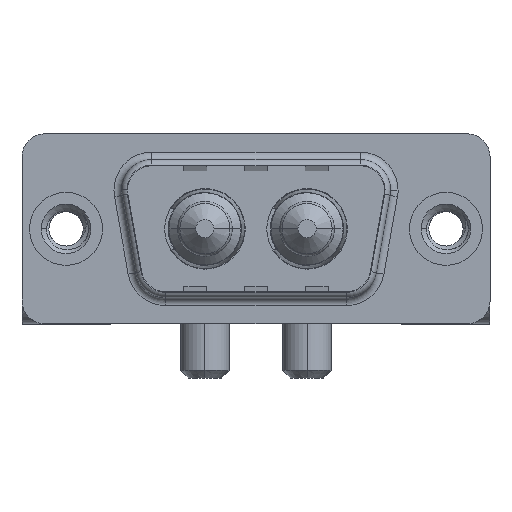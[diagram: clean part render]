
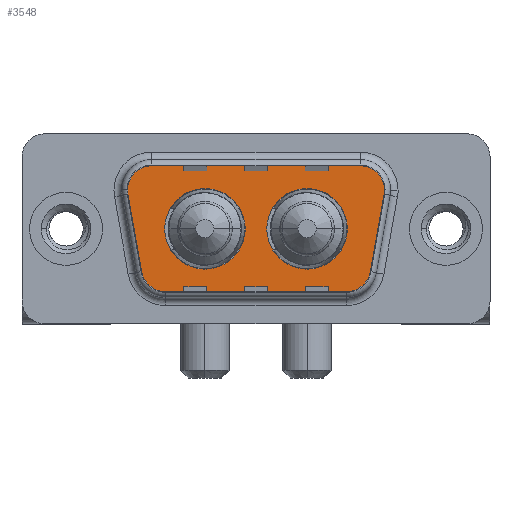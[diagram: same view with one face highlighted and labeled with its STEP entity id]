
A CAD part, top view. The second image highlights one B-rep face of the part: STEP entity #3548.
In plain terms, the highlighted planar face has unit normal (0, 0, 1).
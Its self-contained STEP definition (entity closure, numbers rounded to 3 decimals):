
#85 = CARTESIAN_POINT ( 'NONE',  ( 9.14, 0., 0. ) ) ;
#160 = ORIENTED_EDGE ( 'NONE', *, *, #9335, .T. ) ;
#173 = CARTESIAN_POINT ( 'NONE',  ( 6.459, -2.9, 0. ) ) ;
#208 = ORIENTED_EDGE ( 'NONE', *, *, #1966, .T. ) ;
#296 = CARTESIAN_POINT ( 'NONE',  ( 18.541, -2.9, 0. ) ) ;
#370 = ORIENTED_EDGE ( 'NONE', *, *, #9653, .T. ) ;
#516 = CARTESIAN_POINT ( 'NONE',  ( 3.466, 2.553, 0. ) ) ;
#538 = LINE ( 'NONE', #2681, #9395 ) ;
#579 = DIRECTION ( 'NONE',  ( 1., 0., 0. ) ) ;
#612 = AXIS2_PLACEMENT_3D ( 'NONE', #296, #8820, #9711 ) ;
#729 = ORIENTED_EDGE ( 'NONE', *, *, #10192, .F. ) ;
#896 = CARTESIAN_POINT ( 'NONE',  ( 19.564, 2.9, 0. ) ) ;
#977 = EDGE_CURVE ( 'NONE', #6027, #11507, #538, .T. ) ;
#1020 = CARTESIAN_POINT ( 'NONE',  ( 5.436, 4.9, 0. ) ) ;
#1031 = CARTESIAN_POINT ( 'NONE',  ( 19.564, 2.9, 0. ) ) ;
#1094 = ORIENTED_EDGE ( 'NONE', *, *, #4804, .F. ) ;
#1356 = DIRECTION ( 'NONE',  ( 1., 0., 0. ) ) ;
#1407 = CIRCLE ( 'NONE', #4452, 2. ) ;
#1592 = VERTEX_POINT ( 'NONE', #5201 ) ;
#1645 = PLANE ( 'NONE',  #7467 ) ;
#1786 = CARTESIAN_POINT ( 'NONE',  ( 5.436, 4.9, 0. ) ) ;
#1832 = DIRECTION ( 'NONE',  ( -1., 0., 0. ) ) ;
#1966 = EDGE_CURVE ( 'NONE', #10022, #3323, #4750, .T. ) ;
#1969 = CARTESIAN_POINT ( 'NONE',  ( 11.79, 0., 0. ) ) ;
#2035 = AXIS2_PLACEMENT_3D ( 'NONE', #9243, #6271, #7282 ) ;
#2036 = DIRECTION ( 'NONE',  ( -1., 0., 0. ) ) ;
#2100 = VERTEX_POINT ( 'NONE', #7900 ) ;
#2272 = VERTEX_POINT ( 'NONE', #10055 ) ;
#2318 = VERTEX_POINT ( 'NONE', #4304 ) ;
#2591 = FACE_BOUND ( 'NONE', #4614, .T. ) ;
#2600 = EDGE_LOOP ( 'NONE', ( #5776, #1094 ) ) ;
#2681 = CARTESIAN_POINT ( 'NONE',  ( 21.534, 2.553, 0. ) ) ;
#2705 = LINE ( 'NONE', #11487, #9283 ) ;
#3005 = DIRECTION ( 'NONE',  ( 0., 0., 1. ) ) ;
#3055 = CIRCLE ( 'NONE', #8319, 2.65 ) ;
#3077 = DIRECTION ( 'NONE',  ( -1., 0., 0. ) ) ;
#3105 = ORIENTED_EDGE ( 'NONE', *, *, #7557, .T. ) ;
#3113 = ORIENTED_EDGE ( 'NONE', *, *, #12267, .T. ) ;
#3160 = ORIENTED_EDGE ( 'NONE', *, *, #11364, .T. ) ;
#3323 = VERTEX_POINT ( 'NONE', #1786 ) ;
#3409 = LINE ( 'NONE', #516, #6702 ) ;
#3548 = ADVANCED_FACE ( 'NONE', ( #8413, #2591, #12083 ), #1645, .T. ) ;
#3656 = AXIS2_PLACEMENT_3D ( 'NONE', #11680, #3005, #6863 ) ;
#3727 = VECTOR ( 'NONE', #8730, 1000. ) ;
#3822 = CIRCLE ( 'NONE', #8668, 2. ) ;
#3905 = DIRECTION ( 'NONE',  ( 0., 0., 1. ) ) ;
#4198 = VERTEX_POINT ( 'NONE', #8765 ) ;
#4213 = EDGE_CURVE ( 'NONE', #10918, #2272, #7889, .T. ) ;
#4224 = EDGE_CURVE ( 'NONE', #5443, #2100, #8508, .T. ) ;
#4304 = CARTESIAN_POINT ( 'NONE',  ( 21.564, 2.9, 0. ) ) ;
#4452 = AXIS2_PLACEMENT_3D ( 'NONE', #5507, #10253, #579 ) ;
#4614 = EDGE_LOOP ( 'NONE', ( #9905, #729 ) ) ;
#4750 = LINE ( 'NONE', #1020, #3727 ) ;
#4804 = EDGE_CURVE ( 'NONE', #2100, #5443, #3055, .T. ) ;
#5037 = CIRCLE ( 'NONE', #612, 2. ) ;
#5201 = CARTESIAN_POINT ( 'NONE',  ( 6.49, 0., 0. ) ) ;
#5383 = CIRCLE ( 'NONE', #5595, 2. ) ;
#5443 = VERTEX_POINT ( 'NONE', #5802 ) ;
#5507 = CARTESIAN_POINT ( 'NONE',  ( 5.436, 2.9, 0. ) ) ;
#5549 = DIRECTION ( 'NONE',  ( 1., 0., 0. ) ) ;
#5595 = AXIS2_PLACEMENT_3D ( 'NONE', #896, #8595, #1832 ) ;
#5776 = ORIENTED_EDGE ( 'NONE', *, *, #4224, .F. ) ;
#5802 = CARTESIAN_POINT ( 'NONE',  ( 18.51, 0., 0. ) ) ;
#6027 = VERTEX_POINT ( 'NONE', #7836 ) ;
#6159 = EDGE_LOOP ( 'NONE', ( #8062, #10809, #3113, #160, #208, #370, #3105, #9988, #3160 ) ) ;
#6271 = DIRECTION ( 'NONE',  ( 0., 0., 1. ) ) ;
#6540 = DIRECTION ( 'NONE',  ( 0.174, 0.985, 0. ) ) ;
#6647 = DIRECTION ( 'NONE',  ( 0., 0., 1. ) ) ;
#6702 = VECTOR ( 'NONE', #11132, 1000. ) ;
#6863 = DIRECTION ( 'NONE',  ( 1., 0., 0. ) ) ;
#7103 = CARTESIAN_POINT ( 'NONE',  ( 15.86, 0., 0. ) ) ;
#7193 = VERTEX_POINT ( 'NONE', #1969 ) ;
#7207 = VERTEX_POINT ( 'NONE', #10690 ) ;
#7209 = EDGE_CURVE ( 'NONE', #7193, #1592, #12160, .T. ) ;
#7282 = DIRECTION ( 'NONE',  ( 1., 0., 0. ) ) ;
#7301 = AXIS2_PLACEMENT_3D ( 'NONE', #85, #6647, #9749 ) ;
#7467 = AXIS2_PLACEMENT_3D ( 'NONE', #11130, #9227, #9358 ) ;
#7557 = EDGE_CURVE ( 'NONE', #4198, #10918, #3409, .T. ) ;
#7836 = CARTESIAN_POINT ( 'NONE',  ( 20.511, -3.247, 0. ) ) ;
#7889 = CIRCLE ( 'NONE', #9105, 2. ) ;
#7900 = CARTESIAN_POINT ( 'NONE',  ( 13.21, 0., 0. ) ) ;
#8062 = ORIENTED_EDGE ( 'NONE', *, *, #11552, .T. ) ;
#8319 = AXIS2_PLACEMENT_3D ( 'NONE', #7103, #10021, #1356 ) ;
#8413 = FACE_BOUND ( 'NONE', #2600, .T. ) ;
#8508 = CIRCLE ( 'NONE', #3656, 2.65 ) ;
#8595 = DIRECTION ( 'NONE',  ( 0., 0., 1. ) ) ;
#8668 = AXIS2_PLACEMENT_3D ( 'NONE', #1031, #11651, #2036 ) ;
#8730 = DIRECTION ( 'NONE',  ( -1., 0., 0. ) ) ;
#8765 = CARTESIAN_POINT ( 'NONE',  ( 3.466, 2.553, 0. ) ) ;
#8820 = DIRECTION ( 'NONE',  ( 0., 0., 1. ) ) ;
#9105 = AXIS2_PLACEMENT_3D ( 'NONE', #173, #3905, #3077 ) ;
#9227 = DIRECTION ( 'NONE',  ( 0., 0., 1. ) ) ;
#9243 = CARTESIAN_POINT ( 'NONE',  ( 9.14, 0., 0. ) ) ;
#9283 = VECTOR ( 'NONE', #5549, 1000. ) ;
#9297 = CIRCLE ( 'NONE', #2035, 2.65 ) ;
#9335 = EDGE_CURVE ( 'NONE', #2318, #10022, #3822, .T. ) ;
#9358 = DIRECTION ( 'NONE',  ( 1., 0., 0. ) ) ;
#9395 = VECTOR ( 'NONE', #6540, 1000. ) ;
#9546 = CARTESIAN_POINT ( 'NONE',  ( 4.489, -3.247, 0. ) ) ;
#9653 = EDGE_CURVE ( 'NONE', #3323, #4198, #1407, .T. ) ;
#9711 = DIRECTION ( 'NONE',  ( 1., 0., 0. ) ) ;
#9749 = DIRECTION ( 'NONE',  ( 1., 0., 0. ) ) ;
#9905 = ORIENTED_EDGE ( 'NONE', *, *, #7209, .F. ) ;
#9988 = ORIENTED_EDGE ( 'NONE', *, *, #4213, .T. ) ;
#10021 = DIRECTION ( 'NONE',  ( 0., 0., 1. ) ) ;
#10022 = VERTEX_POINT ( 'NONE', #11908 ) ;
#10055 = CARTESIAN_POINT ( 'NONE',  ( 6.459, -4.9, 0. ) ) ;
#10192 = EDGE_CURVE ( 'NONE', #1592, #7193, #9297, .T. ) ;
#10253 = DIRECTION ( 'NONE',  ( 0., 0., 1. ) ) ;
#10690 = CARTESIAN_POINT ( 'NONE',  ( 18.541, -4.9, 0. ) ) ;
#10809 = ORIENTED_EDGE ( 'NONE', *, *, #977, .T. ) ;
#10918 = VERTEX_POINT ( 'NONE', #9546 ) ;
#11130 = CARTESIAN_POINT ( 'NONE',  ( 18.541, -2.9, 0. ) ) ;
#11132 = DIRECTION ( 'NONE',  ( 0.174, -0.985, 0. ) ) ;
#11364 = EDGE_CURVE ( 'NONE', #2272, #7207, #2705, .T. ) ;
#11487 = CARTESIAN_POINT ( 'NONE',  ( 6.459, -4.9, 0. ) ) ;
#11507 = VERTEX_POINT ( 'NONE', #11809 ) ;
#11552 = EDGE_CURVE ( 'NONE', #7207, #6027, #5037, .T. ) ;
#11651 = DIRECTION ( 'NONE',  ( 0., 0., 1. ) ) ;
#11680 = CARTESIAN_POINT ( 'NONE',  ( 15.86, 0., 0. ) ) ;
#11809 = CARTESIAN_POINT ( 'NONE',  ( 21.534, 2.553, 0. ) ) ;
#11908 = CARTESIAN_POINT ( 'NONE',  ( 19.564, 4.9, 0. ) ) ;
#12083 = FACE_OUTER_BOUND ( 'NONE', #6159, .T. ) ;
#12160 = CIRCLE ( 'NONE', #7301, 2.65 ) ;
#12267 = EDGE_CURVE ( 'NONE', #11507, #2318, #5383, .T. ) ;
